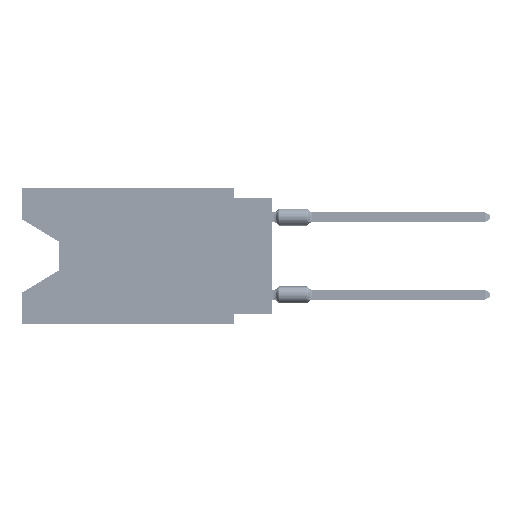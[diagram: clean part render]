
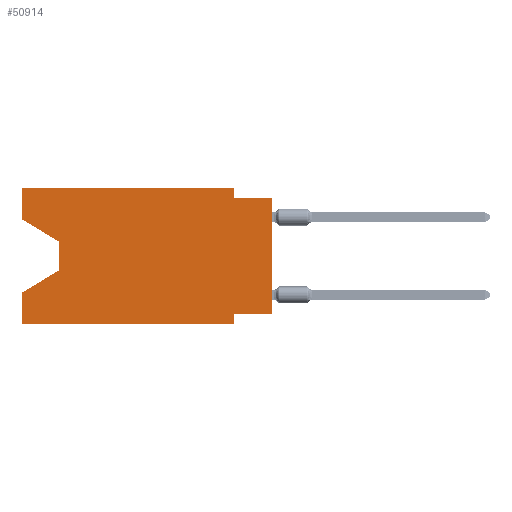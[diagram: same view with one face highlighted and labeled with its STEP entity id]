
A CAD part, left-side view. The second image highlights one B-rep face of the part: STEP entity #50914.
In plain terms, the highlighted planar face has unit normal (-1, 0, 0).
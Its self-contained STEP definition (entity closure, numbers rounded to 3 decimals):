
#83 = CARTESIAN_POINT ( 'NONE',  ( 0., 0., 0. ) ) ;
#733 = VECTOR ( 'NONE', #76822, 1000. ) ;
#1746 = VECTOR ( 'NONE', #40944, 1000. ) ;
#4510 = VECTOR ( 'NONE', #83386, 1000. ) ;
#5262 = PLANE ( 'NONE',  #84216 ) ;
#6083 = VECTOR ( 'NONE', #70282, 1000. ) ;
#10185 = CARTESIAN_POINT ( 'NONE',  ( 0., 2.54, -8.89 ) ) ;
#12098 = VERTEX_POINT ( 'NONE', #22988 ) ;
#14232 = DIRECTION ( 'NONE',  ( 0., -1., 0. ) ) ;
#17302 = DIRECTION ( 'NONE',  ( 0., 0., -1. ) ) ;
#17676 = CARTESIAN_POINT ( 'NONE',  ( 0., 16.383, 0. ) ) ;
#17735 = DIRECTION ( 'NONE',  ( 0., 0., -1. ) ) ;
#18572 = CARTESIAN_POINT ( 'NONE',  ( 0., 16.383, -2.038 ) ) ;
#19608 = CARTESIAN_POINT ( 'NONE',  ( 0., 16.383, -8.89 ) ) ;
#19693 = VECTOR ( 'NONE', #64042, 1000. ) ;
#19921 = CARTESIAN_POINT ( 'NONE',  ( 0., 16.383, 0. ) ) ;
#21988 = VECTOR ( 'NONE', #87076, 1000. ) ;
#22643 = CARTESIAN_POINT ( 'NONE',  ( 0., 2.54, 0. ) ) ;
#22729 = LINE ( 'NONE', #83543, #1746 ) ;
#22988 = CARTESIAN_POINT ( 'NONE',  ( 0., 2.54, 0. ) ) ;
#23364 = EDGE_CURVE ( 'NONE', #65726, #24854, #37620, .T. ) ;
#24854 = VERTEX_POINT ( 'NONE', #42442 ) ;
#25099 = CARTESIAN_POINT ( 'NONE',  ( 0., 0., -8.255 ) ) ;
#25702 = LINE ( 'NONE', #19921, #83267 ) ;
#27301 = EDGE_CURVE ( 'NONE', #63703, #24854, #22729, .T. ) ;
#28383 = CARTESIAN_POINT ( 'NONE',  ( 0., 2.54, -8.89 ) ) ;
#28583 = LINE ( 'NONE', #56096, #6083 ) ;
#29024 = EDGE_CURVE ( 'NONE', #55229, #35535, #50583, .T. ) ;
#29352 = EDGE_CURVE ( 'NONE', #44391, #55229, #85914, .T. ) ;
#35535 = VERTEX_POINT ( 'NONE', #28383 ) ;
#35861 = VERTEX_POINT ( 'NONE', #18572 ) ;
#35983 = LINE ( 'NONE', #75089, #77430 ) ;
#36923 = VECTOR ( 'NONE', #14232, 1000. ) ;
#37620 = LINE ( 'NONE', #17676, #4510 ) ;
#39455 = CARTESIAN_POINT ( 'NONE',  ( 0., 0., -0.635 ) ) ;
#39571 = LINE ( 'NONE', #19608, #21988 ) ;
#40944 = DIRECTION ( 'NONE',  ( 0., 0.855, -0.519 ) ) ;
#41305 = CARTESIAN_POINT ( 'NONE',  ( 0., 16.383, 0. ) ) ;
#41348 = DIRECTION ( 'NONE',  ( 0., -0.855, -0.519 ) ) ;
#42442 = CARTESIAN_POINT ( 'NONE',  ( 0., 16.383, -6.852 ) ) ;
#43354 = EDGE_CURVE ( 'NONE', #44391, #52937, #74231, .T. ) ;
#43606 = LINE ( 'NONE', #56069, #19693 ) ;
#44391 = VERTEX_POINT ( 'NONE', #64083 ) ;
#47685 = EDGE_CURVE ( 'NONE', #48344, #63703, #43606, .T. ) ;
#48344 = VERTEX_POINT ( 'NONE', #60763 ) ;
#49357 = ORIENTED_EDGE ( 'NONE', *, *, #70366, .F. ) ;
#50583 = LINE ( 'NONE', #10185, #82036 ) ;
#50826 = CARTESIAN_POINT ( 'NONE',  ( 0., 2.54, -0.635 ) ) ;
#50914 = ADVANCED_FACE ( 'NONE', ( #66085 ), #5262, .F. ) ;
#52812 = EDGE_CURVE ( 'NONE', #12098, #66035, #83467, .T. ) ;
#52937 = VERTEX_POINT ( 'NONE', #39455 ) ;
#53827 = ORIENTED_EDGE ( 'NONE', *, *, #23364, .F. ) ;
#54904 = ORIENTED_EDGE ( 'NONE', *, *, #27301, .T. ) ;
#55146 = EDGE_CURVE ( 'NONE', #66035, #52937, #28583, .T. ) ;
#55229 = VERTEX_POINT ( 'NONE', #58877 ) ;
#56069 = CARTESIAN_POINT ( 'NONE',  ( 0., 13.97, -3.505 ) ) ;
#56096 = CARTESIAN_POINT ( 'NONE',  ( 0., 0., -0.635 ) ) ;
#58424 = DIRECTION ( 'NONE',  ( 0., 1., 0. ) ) ;
#58813 = ORIENTED_EDGE ( 'NONE', *, *, #43354, .T. ) ;
#58877 = CARTESIAN_POINT ( 'NONE',  ( 0., 2.54, -8.255 ) ) ;
#59339 = CARTESIAN_POINT ( 'NONE',  ( 0., 16.383, -8.89 ) ) ;
#59541 = CARTESIAN_POINT ( 'NONE',  ( 0., 13.97, -5.385 ) ) ;
#60763 = CARTESIAN_POINT ( 'NONE',  ( 0., 13.97, -3.505 ) ) ;
#61112 = ORIENTED_EDGE ( 'NONE', *, *, #76415, .F. ) ;
#63167 = VERTEX_POINT ( 'NONE', #71520 ) ;
#63703 = VERTEX_POINT ( 'NONE', #59541 ) ;
#64042 = DIRECTION ( 'NONE',  ( 0., 0., -1. ) ) ;
#64083 = CARTESIAN_POINT ( 'NONE',  ( 0., 0., -8.255 ) ) ;
#65214 = DIRECTION ( 'NONE',  ( 1., 0., 0. ) ) ;
#65486 = ORIENTED_EDGE ( 'NONE', *, *, #47685, .T. ) ;
#65726 = VERTEX_POINT ( 'NONE', #59339 ) ;
#66035 = VERTEX_POINT ( 'NONE', #50826 ) ;
#66085 = FACE_OUTER_BOUND ( 'NONE', #76940, .T. ) ;
#66348 = ORIENTED_EDGE ( 'NONE', *, *, #55146, .F. ) ;
#67506 = LINE ( 'NONE', #41305, #36923 ) ;
#67840 = DIRECTION ( 'NONE',  ( 0., 0., 1. ) ) ;
#70282 = DIRECTION ( 'NONE',  ( 0., -1., 0. ) ) ;
#70366 = EDGE_CURVE ( 'NONE', #35861, #63167, #25702, .T. ) ;
#71021 = ORIENTED_EDGE ( 'NONE', *, *, #29352, .F. ) ;
#71520 = CARTESIAN_POINT ( 'NONE',  ( 0., 16.383, 0. ) ) ;
#74231 = LINE ( 'NONE', #83, #83816 ) ;
#74455 = ORIENTED_EDGE ( 'NONE', *, *, #83915, .T. ) ;
#75089 = CARTESIAN_POINT ( 'NONE',  ( 0., 16.383, -2.038 ) ) ;
#76415 = EDGE_CURVE ( 'NONE', #63167, #12098, #67506, .T. ) ;
#76822 = DIRECTION ( 'NONE',  ( 0., 0., -1. ) ) ;
#76940 = EDGE_LOOP ( 'NONE', ( #87084, #65486, #54904, #53827, #74455, #80806, #71021, #58813, #66348, #79117, #61112, #49357 ) ) ;
#77430 = VECTOR ( 'NONE', #41348, 1000. ) ;
#79117 = ORIENTED_EDGE ( 'NONE', *, *, #52812, .F. ) ;
#79328 = VECTOR ( 'NONE', #58424, 1000. ) ;
#80806 = ORIENTED_EDGE ( 'NONE', *, *, #29024, .F. ) ;
#81338 = DIRECTION ( 'NONE',  ( 0., 0., 1. ) ) ;
#82036 = VECTOR ( 'NONE', #17302, 1000. ) ;
#83267 = VECTOR ( 'NONE', #67840, 1000. ) ;
#83386 = DIRECTION ( 'NONE',  ( 0., 0., 1. ) ) ;
#83467 = LINE ( 'NONE', #22643, #733 ) ;
#83543 = CARTESIAN_POINT ( 'NONE',  ( 0., 13.97, -5.385 ) ) ;
#83816 = VECTOR ( 'NONE', #81338, 1000. ) ;
#83915 = EDGE_CURVE ( 'NONE', #65726, #35535, #39571, .T. ) ;
#84216 = AXIS2_PLACEMENT_3D ( 'NONE', #86059, #65214, #17735 ) ;
#85267 = EDGE_CURVE ( 'NONE', #35861, #48344, #35983, .T. ) ;
#85914 = LINE ( 'NONE', #25099, #79328 ) ;
#86059 = CARTESIAN_POINT ( 'NONE',  ( 0., 16.383, 0. ) ) ;
#87076 = DIRECTION ( 'NONE',  ( 0., -1., 0. ) ) ;
#87084 = ORIENTED_EDGE ( 'NONE', *, *, #85267, .T. ) ;
